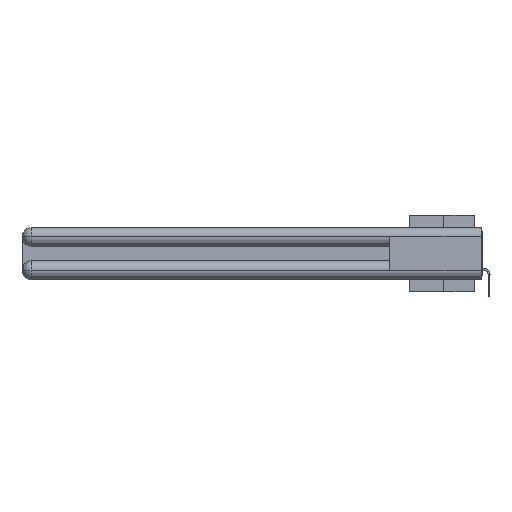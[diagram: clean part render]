
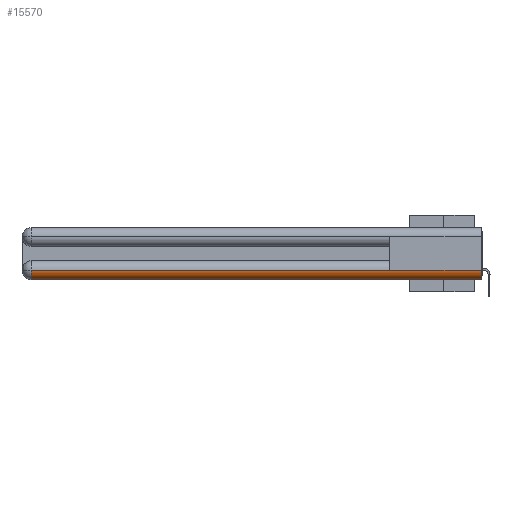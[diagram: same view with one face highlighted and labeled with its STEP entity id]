
A CAD part, left-side view. The second image highlights one B-rep face of the part: STEP entity #15570.
In plain terms, the highlighted cylindrical face has radius 1.562 mm (diameter 3.124 mm), a partial arc.
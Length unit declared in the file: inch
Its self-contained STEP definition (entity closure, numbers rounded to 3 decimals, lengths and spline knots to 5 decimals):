
#1159 = DIRECTION ( 'NONE',  ( 0., 1., 0. ) ) ;
#1165 = VERTEX_POINT ( 'NONE', #15974 ) ;
#1495 = VERTEX_POINT ( 'NONE', #4849 ) ;
#3797 = DIRECTION ( 'NONE',  ( 0., -1., 0. ) ) ;
#4659 = EDGE_CURVE ( 'NONE', #1165, #34448, #33823, .T. ) ;
#4669 = CYLINDRICAL_SURFACE ( 'NONE', #18012, 0.0615 ) ;
#4795 = DIRECTION ( 'NONE',  ( 0., -1., 0. ) ) ;
#4836 = FACE_OUTER_BOUND ( 'NONE', #25882, .T. ) ;
#4849 = CARTESIAN_POINT ( 'NONE',  ( 0.0615, 0., -0.34 ) ) ;
#5189 = CARTESIAN_POINT ( 'NONE',  ( 0.0615, 2.94, -0.2785 ) ) ;
#6142 = ORIENTED_EDGE ( 'NONE', *, *, #23344, .T. ) ;
#7896 = CARTESIAN_POINT ( 'NONE',  ( 0., 2.94, -0.2785 ) ) ;
#8430 = LINE ( 'NONE', #24284, #12306 ) ;
#10174 = ORIENTED_EDGE ( 'NONE', *, *, #18124, .F. ) ;
#12069 = AXIS2_PLACEMENT_3D ( 'NONE', #17329, #3797, #25539 ) ;
#12306 = VECTOR ( 'NONE', #27469, 39.37008 ) ;
#13223 = DIRECTION ( 'NONE',  ( 0., 0., -1. ) ) ;
#13506 = VERTEX_POINT ( 'NONE', #26474 ) ;
#13711 = ORIENTED_EDGE ( 'NONE', *, *, #32272, .F. ) ;
#15570 = ADVANCED_FACE ( 'NONE', ( #4836 ), #4669, .T. ) ;
#15660 = LINE ( 'NONE', #18347, #28386 ) ;
#15974 = CARTESIAN_POINT ( 'NONE',  ( 0., 0.6, -0.2785 ) ) ;
#16301 = ORIENTED_EDGE ( 'NONE', *, *, #24556, .F. ) ;
#17329 = CARTESIAN_POINT ( 'NONE',  ( 0.0615, 0., -0.2785 ) ) ;
#18012 = AXIS2_PLACEMENT_3D ( 'NONE', #23565, #31687, #13223 ) ;
#18124 = EDGE_CURVE ( 'NONE', #1165, #34923, #15660, .T. ) ;
#18347 = CARTESIAN_POINT ( 'NONE',  ( 0., 0., -0.2785 ) ) ;
#22316 = CIRCLE ( 'NONE', #12069, 0.0615 ) ;
#23117 = ORIENTED_EDGE ( 'NONE', *, *, #4659, .T. ) ;
#23344 = EDGE_CURVE ( 'NONE', #34448, #13506, #31271, .T. ) ;
#23565 = CARTESIAN_POINT ( 'NONE',  ( 0.0615, 0., -0.2785 ) ) ;
#24284 = CARTESIAN_POINT ( 'NONE',  ( 0.0615, 0., -0.34 ) ) ;
#24556 = EDGE_CURVE ( 'NONE', #34923, #1495, #22316, .T. ) ;
#25195 = CARTESIAN_POINT ( 'NONE',  ( 0., 0., -0.2785 ) ) ;
#25539 = DIRECTION ( 'NONE',  ( 1., 0., 0. ) ) ;
#25882 = EDGE_LOOP ( 'NONE', ( #23117, #6142, #13711, #16301, #10174 ) ) ;
#26215 = AXIS2_PLACEMENT_3D ( 'NONE', #5189, #26572, #34859 ) ;
#26474 = CARTESIAN_POINT ( 'NONE',  ( 0.0615, 2.94, -0.34 ) ) ;
#26551 = CARTESIAN_POINT ( 'NONE',  ( 0., 0., -0.2785 ) ) ;
#26572 = DIRECTION ( 'NONE',  ( 0., -1., 0. ) ) ;
#27469 = DIRECTION ( 'NONE',  ( 0., 1., 0. ) ) ;
#28386 = VECTOR ( 'NONE', #4795, 39.37008 ) ;
#31271 = CIRCLE ( 'NONE', #26215, 0.0615 ) ;
#31592 = VECTOR ( 'NONE', #1159, 39.37008 ) ;
#31687 = DIRECTION ( 'NONE',  ( 0., -1., 0. ) ) ;
#32272 = EDGE_CURVE ( 'NONE', #1495, #13506, #8430, .T. ) ;
#33823 = LINE ( 'NONE', #25195, #31592 ) ;
#34448 = VERTEX_POINT ( 'NONE', #7896 ) ;
#34859 = DIRECTION ( 'NONE',  ( 0., 0., 1. ) ) ;
#34923 = VERTEX_POINT ( 'NONE', #26551 ) ;
